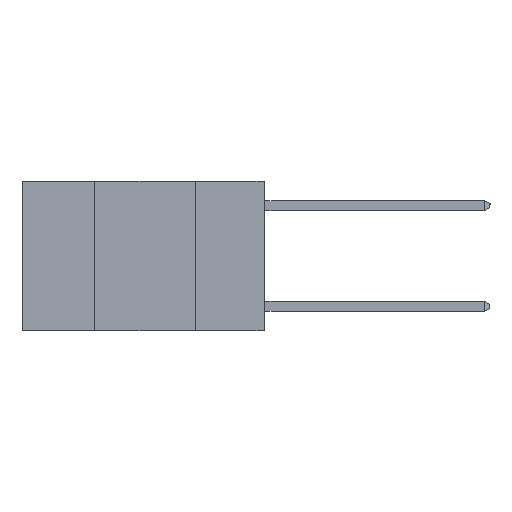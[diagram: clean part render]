
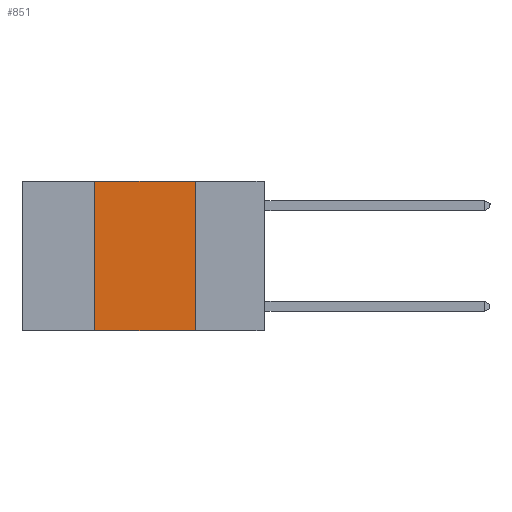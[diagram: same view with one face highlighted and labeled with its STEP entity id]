
A CAD part, left-side view. The second image highlights one B-rep face of the part: STEP entity #851.
In plain terms, the highlighted planar face has unit normal (-1, 0, 0).
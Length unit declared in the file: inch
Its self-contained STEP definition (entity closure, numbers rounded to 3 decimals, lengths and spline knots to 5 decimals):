
#165 = CARTESIAN_POINT ( 'NONE',  ( 0., 0.17, -0.37 ) ) ;
#851 = ADVANCED_FACE ( 'NONE', ( #3496 ), #8972, .F. ) ;
#900 = LINE ( 'NONE', #5139, #9014 ) ;
#1057 = CARTESIAN_POINT ( 'NONE',  ( 0., 0.42, 0. ) ) ;
#1101 = VERTEX_POINT ( 'NONE', #1057 ) ;
#1163 = DIRECTION ( 'NONE',  ( 0., 0., 1. ) ) ;
#1294 = EDGE_CURVE ( 'NONE', #4724, #2826, #5638, .T. ) ;
#1445 = EDGE_CURVE ( 'NONE', #5144, #2826, #9780, .T. ) ;
#1449 = EDGE_CURVE ( 'NONE', #1101, #4724, #8109, .T. ) ;
#1639 = CARTESIAN_POINT ( 'NONE',  ( 0., 0.6, 0. ) ) ;
#1659 = EDGE_CURVE ( 'NONE', #5144, #1101, #900, .T. ) ;
#1834 = VECTOR ( 'NONE', #7725, 39.37008 ) ;
#2826 = VERTEX_POINT ( 'NONE', #165 ) ;
#3496 = FACE_OUTER_BOUND ( 'NONE', #8957, .T. ) ;
#3583 = CARTESIAN_POINT ( 'NONE',  ( 0., 0.17, 0. ) ) ;
#3593 = AXIS2_PLACEMENT_3D ( 'NONE', #4295, #8898, #8628 ) ;
#4295 = CARTESIAN_POINT ( 'NONE',  ( 0., 0.6, 0. ) ) ;
#4724 = VERTEX_POINT ( 'NONE', #3583 ) ;
#4811 = DIRECTION ( 'NONE',  ( 0., -1., 0. ) ) ;
#5139 = CARTESIAN_POINT ( 'NONE',  ( 0., 0.42, 0. ) ) ;
#5144 = VERTEX_POINT ( 'NONE', #9109 ) ;
#5638 = LINE ( 'NONE', #7540, #9258 ) ;
#7416 = ORIENTED_EDGE ( 'NONE', *, *, #1294, .F. ) ;
#7540 = CARTESIAN_POINT ( 'NONE',  ( 0., 0.17, 0. ) ) ;
#7556 = ORIENTED_EDGE ( 'NONE', *, *, #1449, .F. ) ;
#7563 = ORIENTED_EDGE ( 'NONE', *, *, #1659, .F. ) ;
#7649 = VECTOR ( 'NONE', #4811, 39.37008 ) ;
#7721 = ORIENTED_EDGE ( 'NONE', *, *, #1445, .T. ) ;
#7725 = DIRECTION ( 'NONE',  ( 0., -1., 0. ) ) ;
#8109 = LINE ( 'NONE', #1639, #7649 ) ;
#8446 = CARTESIAN_POINT ( 'NONE',  ( 0., 0.6, -0.37 ) ) ;
#8628 = DIRECTION ( 'NONE',  ( 0., 0., -1. ) ) ;
#8898 = DIRECTION ( 'NONE',  ( 1., 0., 0. ) ) ;
#8957 = EDGE_LOOP ( 'NONE', ( #7416, #7556, #7563, #7721 ) ) ;
#8972 = PLANE ( 'NONE',  #3593 ) ;
#9001 = DIRECTION ( 'NONE',  ( 0., 0., -1. ) ) ;
#9014 = VECTOR ( 'NONE', #1163, 39.37008 ) ;
#9109 = CARTESIAN_POINT ( 'NONE',  ( 0., 0.42, -0.37 ) ) ;
#9258 = VECTOR ( 'NONE', #9001, 39.37008 ) ;
#9780 = LINE ( 'NONE', #8446, #1834 ) ;
